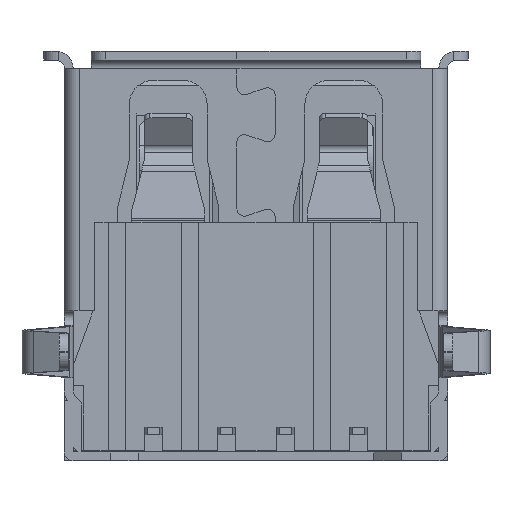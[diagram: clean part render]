
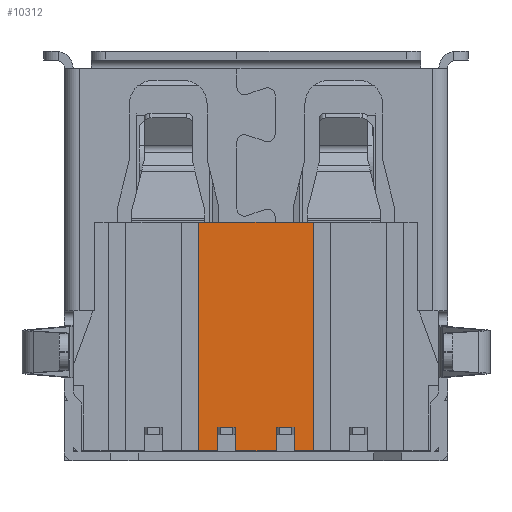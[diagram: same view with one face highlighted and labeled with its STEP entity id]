
A CAD part, front view. The second image highlights one B-rep face of the part: STEP entity #10312.
In plain terms, the highlighted planar face has unit normal (0, -1, 0).
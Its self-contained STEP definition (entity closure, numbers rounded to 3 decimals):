
#413 = LINE ( 'NONE', #14665, #556 ) ;
#433 = DIRECTION ( 'NONE',  ( 0., -1., 0. ) ) ;
#556 = VECTOR ( 'NONE', #9577, 1000. ) ;
#657 = FACE_OUTER_BOUND ( 'NONE', #22241, .T. ) ;
#704 = EDGE_CURVE ( 'NONE', #5682, #4925, #834, .T. ) ;
#779 = LINE ( 'NONE', #20569, #16081 ) ;
#834 = LINE ( 'NONE', #13327, #9277 ) ;
#1241 = EDGE_CURVE ( 'NONE', #13264, #9184, #22699, .T. ) ;
#1286 = VERTEX_POINT ( 'NONE', #6551 ) ;
#1474 = VERTEX_POINT ( 'NONE', #17234 ) ;
#2787 = EDGE_CURVE ( 'NONE', #1474, #1286, #779, .T. ) ;
#3097 = EDGE_CURVE ( 'NONE', #12580, #15242, #20047, .T. ) ;
#3238 = DIRECTION ( 'NONE',  ( -1., 0., 0. ) ) ;
#3451 = ORIENTED_EDGE ( 'NONE', *, *, #3097, .F. ) ;
#3647 = CARTESIAN_POINT ( 'NONE',  ( 0., -6.1, -3.98 ) ) ;
#3790 = LINE ( 'NONE', #11002, #21271 ) ;
#4147 = ORIENTED_EDGE ( 'NONE', *, *, #2787, .T. ) ;
#4272 = ORIENTED_EDGE ( 'NONE', *, *, #19743, .T. ) ;
#4837 = ORIENTED_EDGE ( 'NONE', *, *, #20861, .T. ) ;
#4925 = VERTEX_POINT ( 'NONE', #8452 ) ;
#5547 = CARTESIAN_POINT ( 'NONE',  ( 0., -6.1, 3.03 ) ) ;
#5682 = VERTEX_POINT ( 'NONE', #22541 ) ;
#5766 = AXIS2_PLACEMENT_3D ( 'NONE', #11037, #433, #14909 ) ;
#5913 = ORIENTED_EDGE ( 'NONE', *, *, #1241, .T. ) ;
#5929 = VECTOR ( 'NONE', #12066, 1000. ) ;
#5954 = DIRECTION ( 'NONE',  ( 0., 0., 1. ) ) ;
#6124 = DIRECTION ( 'NONE',  ( 0., 0., -1. ) ) ;
#6551 = CARTESIAN_POINT ( 'NONE',  ( 4.95, -6.1, -3.98 ) ) ;
#7283 = ORIENTED_EDGE ( 'NONE', *, *, #704, .T. ) ;
#7312 = DIRECTION ( 'NONE',  ( 0., 0., -1. ) ) ;
#7554 = VECTOR ( 'NONE', #10863, 1000. ) ;
#8053 = CARTESIAN_POINT ( 'NONE',  ( 0., -6.1, -4.77 ) ) ;
#8391 = LINE ( 'NONE', #10975, #5929 ) ;
#8452 = CARTESIAN_POINT ( 'NONE',  ( 5.55, -6.1, -4.77 ) ) ;
#9030 = VECTOR ( 'NONE', #7312, 1000. ) ;
#9184 = VERTEX_POINT ( 'NONE', #18560 ) ;
#9277 = VECTOR ( 'NONE', #6124, 1000. ) ;
#9577 = DIRECTION ( 'NONE',  ( 0., 0., -1. ) ) ;
#9601 = ORIENTED_EDGE ( 'NONE', *, *, #16571, .T. ) ;
#9612 = VERTEX_POINT ( 'NONE', #20751 ) ;
#10262 = DIRECTION ( 'NONE',  ( 1., 0., 0. ) ) ;
#10312 = ADVANCED_FACE ( 'NONE', ( #657 ), #20324, .T. ) ;
#10863 = DIRECTION ( 'NONE',  ( 1., 0., 0. ) ) ;
#10975 = CARTESIAN_POINT ( 'NONE',  ( 0., -6.1, -4.77 ) ) ;
#11002 = CARTESIAN_POINT ( 'NONE',  ( 8.2, -6.1, 0. ) ) ;
#11037 = CARTESIAN_POINT ( 'NONE',  ( 0., -6.1, 0. ) ) ;
#11722 = DIRECTION ( 'NONE',  ( -1., 0., 0. ) ) ;
#12066 = DIRECTION ( 'NONE',  ( -1., 0., 0. ) ) ;
#12219 = LINE ( 'NONE', #23039, #18435 ) ;
#12336 = CARTESIAN_POINT ( 'NONE',  ( 6.95, -6.1, -4.77 ) ) ;
#12449 = EDGE_CURVE ( 'NONE', #13264, #4925, #8391, .T. ) ;
#12580 = VERTEX_POINT ( 'NONE', #14847 ) ;
#12634 = VECTOR ( 'NONE', #22932, 1000. ) ;
#12870 = LINE ( 'NONE', #18051, #9030 ) ;
#13264 = VERTEX_POINT ( 'NONE', #12336 ) ;
#13327 = CARTESIAN_POINT ( 'NONE',  ( 5.55, -6.1, -3.98 ) ) ;
#13567 = VECTOR ( 'NONE', #11722, 1000. ) ;
#13569 = LINE ( 'NONE', #20629, #14142 ) ;
#13782 = ORIENTED_EDGE ( 'NONE', *, *, #22967, .F. ) ;
#14142 = VECTOR ( 'NONE', #10262, 1000. ) ;
#14579 = ORIENTED_EDGE ( 'NONE', *, *, #12449, .F. ) ;
#14665 = CARTESIAN_POINT ( 'NONE',  ( 7.55, -6.1, -3.98 ) ) ;
#14847 = CARTESIAN_POINT ( 'NONE',  ( 4.3, -6.1, 3.03 ) ) ;
#14859 = EDGE_CURVE ( 'NONE', #19547, #21941, #413, .T. ) ;
#14909 = DIRECTION ( 'NONE',  ( -1., 0., 0. ) ) ;
#15242 = VERTEX_POINT ( 'NONE', #21166 ) ;
#15385 = ORIENTED_EDGE ( 'NONE', *, *, #14859, .T. ) ;
#15639 = CARTESIAN_POINT ( 'NONE',  ( 6.95, -6.1, -4.77 ) ) ;
#16081 = VECTOR ( 'NONE', #5954, 1000. ) ;
#16100 = VECTOR ( 'NONE', #21814, 1000. ) ;
#16571 = EDGE_CURVE ( 'NONE', #1286, #5682, #13569, .T. ) ;
#17121 = ORIENTED_EDGE ( 'NONE', *, *, #19112, .F. ) ;
#17234 = CARTESIAN_POINT ( 'NONE',  ( 4.95, -6.1, -4.77 ) ) ;
#17928 = LINE ( 'NONE', #3647, #7554 ) ;
#17981 = CARTESIAN_POINT ( 'NONE',  ( 7.55, -6.1, -4.77 ) ) ;
#18051 = CARTESIAN_POINT ( 'NONE',  ( 4.3, -6.1, 0. ) ) ;
#18261 = ORIENTED_EDGE ( 'NONE', *, *, #22268, .T. ) ;
#18435 = VECTOR ( 'NONE', #3238, 1000. ) ;
#18560 = CARTESIAN_POINT ( 'NONE',  ( 6.95, -6.1, -3.98 ) ) ;
#19112 = EDGE_CURVE ( 'NONE', #1474, #20314, #20777, .T. ) ;
#19547 = VERTEX_POINT ( 'NONE', #22984 ) ;
#19743 = EDGE_CURVE ( 'NONE', #9184, #19547, #17928, .T. ) ;
#19939 = DIRECTION ( 'NONE',  ( 0., 0., 1. ) ) ;
#20047 = LINE ( 'NONE', #5547, #16100 ) ;
#20314 = VERTEX_POINT ( 'NONE', #21158 ) ;
#20324 = PLANE ( 'NONE',  #5766 ) ;
#20569 = CARTESIAN_POINT ( 'NONE',  ( 4.95, -6.1, -4.77 ) ) ;
#20629 = CARTESIAN_POINT ( 'NONE',  ( 0., -6.1, -3.98 ) ) ;
#20751 = CARTESIAN_POINT ( 'NONE',  ( 8.2, -6.1, -4.77 ) ) ;
#20777 = LINE ( 'NONE', #8053, #13567 ) ;
#20861 = EDGE_CURVE ( 'NONE', #12580, #20314, #12870, .T. ) ;
#21158 = CARTESIAN_POINT ( 'NONE',  ( 4.3, -6.1, -4.77 ) ) ;
#21166 = CARTESIAN_POINT ( 'NONE',  ( 8.2, -6.1, 3.03 ) ) ;
#21271 = VECTOR ( 'NONE', #19939, 1000. ) ;
#21814 = DIRECTION ( 'NONE',  ( 1., 0., 0. ) ) ;
#21941 = VERTEX_POINT ( 'NONE', #17981 ) ;
#22241 = EDGE_LOOP ( 'NONE', ( #5913, #4272, #15385, #13782, #18261, #3451, #4837, #17121, #4147, #9601, #7283, #14579 ) ) ;
#22268 = EDGE_CURVE ( 'NONE', #9612, #15242, #3790, .T. ) ;
#22541 = CARTESIAN_POINT ( 'NONE',  ( 5.55, -6.1, -3.98 ) ) ;
#22699 = LINE ( 'NONE', #15639, #12634 ) ;
#22932 = DIRECTION ( 'NONE',  ( 0., 0., 1. ) ) ;
#22967 = EDGE_CURVE ( 'NONE', #9612, #21941, #12219, .T. ) ;
#22984 = CARTESIAN_POINT ( 'NONE',  ( 7.55, -6.1, -3.98 ) ) ;
#23039 = CARTESIAN_POINT ( 'NONE',  ( 0., -6.1, -4.77 ) ) ;
